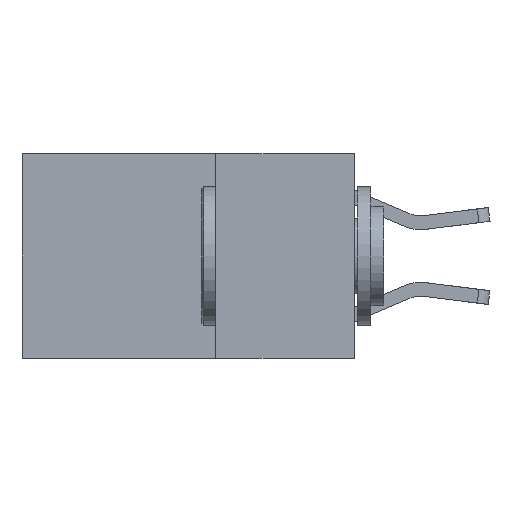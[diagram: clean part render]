
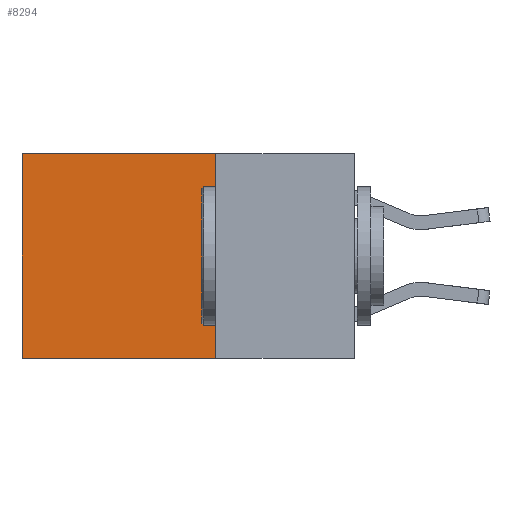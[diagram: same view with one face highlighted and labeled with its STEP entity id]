
A CAD part, left-side view. The second image highlights one B-rep face of the part: STEP entity #8294.
In plain terms, the highlighted planar face has unit normal (-1, 0, 0).
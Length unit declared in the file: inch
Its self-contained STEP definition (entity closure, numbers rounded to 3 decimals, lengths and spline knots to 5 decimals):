
#136 = VECTOR ( 'NONE', #4858, 39.37008 ) ;
#485 = CARTESIAN_POINT ( 'NONE',  ( 0.2625, 0.25, -0.37 ) ) ;
#504 = ORIENTED_EDGE ( 'NONE', *, *, #5715, .F. ) ;
#1054 = DIRECTION ( 'NONE',  ( 0., 1., 0. ) ) ;
#1492 = EDGE_CURVE ( 'NONE', #1858, #3514, #3650, .T. ) ;
#1594 = DIRECTION ( 'NONE',  ( 0., 0., -1. ) ) ;
#1715 = ORIENTED_EDGE ( 'NONE', *, *, #6460, .T. ) ;
#1858 = VERTEX_POINT ( 'NONE', #11120 ) ;
#2049 = AXIS2_PLACEMENT_3D ( 'NONE', #5991, #6861, #1594 ) ;
#2431 = EDGE_CURVE ( 'NONE', #1858, #4264, #7479, .T. ) ;
#2565 = LINE ( 'NONE', #10156, #136 ) ;
#2926 = DIRECTION ( 'NONE',  ( 0., 1., 0. ) ) ;
#2964 = CARTESIAN_POINT ( 'NONE',  ( 0.2625, 0.25, 0. ) ) ;
#3006 = CARTESIAN_POINT ( 'NONE',  ( 0.2625, 0.6, -0.37 ) ) ;
#3514 = VERTEX_POINT ( 'NONE', #9004 ) ;
#3570 = EDGE_LOOP ( 'NONE', ( #1715, #504, #7731, #6703 ) ) ;
#3650 = LINE ( 'NONE', #2964, #8037 ) ;
#4264 = VERTEX_POINT ( 'NONE', #485 ) ;
#4702 = FACE_OUTER_BOUND ( 'NONE', #3570, .T. ) ;
#4858 = DIRECTION ( 'NONE',  ( 0., 0., -1. ) ) ;
#4910 = CARTESIAN_POINT ( 'NONE',  ( 0.2625, 0.25, 0. ) ) ;
#5085 = PLANE ( 'NONE',  #2049 ) ;
#5715 = EDGE_CURVE ( 'NONE', #4264, #5812, #10008, .T. ) ;
#5806 = DIRECTION ( 'NONE',  ( 0., 0., -1. ) ) ;
#5812 = VERTEX_POINT ( 'NONE', #3006 ) ;
#5991 = CARTESIAN_POINT ( 'NONE',  ( 0.2625, 0.25, 0. ) ) ;
#6460 = EDGE_CURVE ( 'NONE', #3514, #5812, #2565, .T. ) ;
#6703 = ORIENTED_EDGE ( 'NONE', *, *, #1492, .T. ) ;
#6861 = DIRECTION ( 'NONE',  ( 1., 0., 0. ) ) ;
#7198 = CARTESIAN_POINT ( 'NONE',  ( 0.2625, 0.25, -0.37 ) ) ;
#7381 = VECTOR ( 'NONE', #1054, 39.37008 ) ;
#7479 = LINE ( 'NONE', #4910, #9542 ) ;
#7731 = ORIENTED_EDGE ( 'NONE', *, *, #2431, .F. ) ;
#8037 = VECTOR ( 'NONE', #2926, 39.37008 ) ;
#8294 = ADVANCED_FACE ( 'NONE', ( #4702 ), #5085, .F. ) ;
#9004 = CARTESIAN_POINT ( 'NONE',  ( 0.2625, 0.6, 0. ) ) ;
#9542 = VECTOR ( 'NONE', #5806, 39.37008 ) ;
#10008 = LINE ( 'NONE', #7198, #7381 ) ;
#10156 = CARTESIAN_POINT ( 'NONE',  ( 0.2625, 0.6, 0. ) ) ;
#11120 = CARTESIAN_POINT ( 'NONE',  ( 0.2625, 0.25, 0. ) ) ;
